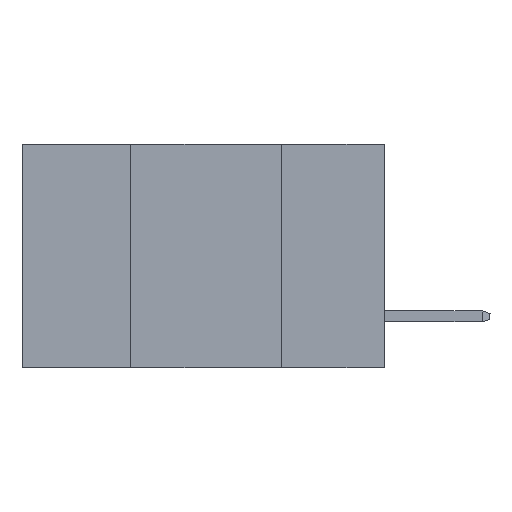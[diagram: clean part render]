
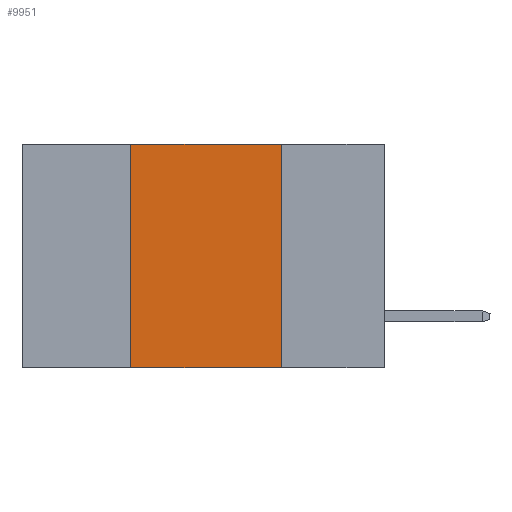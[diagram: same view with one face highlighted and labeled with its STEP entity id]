
A CAD part, left-side view. The second image highlights one B-rep face of the part: STEP entity #9951.
In plain terms, the highlighted planar face has unit normal (-1, 0, 0).
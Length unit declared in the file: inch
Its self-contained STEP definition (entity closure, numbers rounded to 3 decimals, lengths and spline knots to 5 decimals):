
#130 = CARTESIAN_POINT ( 'NONE',  ( 0., 0.17, -0.37 ) ) ;
#491 = DIRECTION ( 'NONE',  ( 0., -1., 0. ) ) ;
#654 = DIRECTION ( 'NONE',  ( 0., 0., 1. ) ) ;
#1088 = VECTOR ( 'NONE', #7853, 39.37008 ) ;
#1345 = VECTOR ( 'NONE', #9363, 39.37008 ) ;
#1347 = VECTOR ( 'NONE', #491, 39.37008 ) ;
#1742 = LINE ( 'NONE', #5525, #1088 ) ;
#1953 = ORIENTED_EDGE ( 'NONE', *, *, #2191, .F. ) ;
#2119 = EDGE_CURVE ( 'NONE', #2372, #7838, #6207, .T. ) ;
#2191 = EDGE_CURVE ( 'NONE', #3699, #8662, #4526, .T. ) ;
#2372 = VERTEX_POINT ( 'NONE', #8064 ) ;
#2835 = CARTESIAN_POINT ( 'NONE',  ( 0., 0.6, -0.37 ) ) ;
#3263 = VECTOR ( 'NONE', #654, 39.37008 ) ;
#3496 = CARTESIAN_POINT ( 'NONE',  ( 0., 0.42, -0.37 ) ) ;
#3699 = VERTEX_POINT ( 'NONE', #3496 ) ;
#3787 = FACE_OUTER_BOUND ( 'NONE', #6253, .T. ) ;
#4526 = LINE ( 'NONE', #7595, #3263 ) ;
#4546 = CARTESIAN_POINT ( 'NONE',  ( 0., 0.6, 0. ) ) ;
#5272 = EDGE_CURVE ( 'NONE', #8662, #2372, #1742, .T. ) ;
#5525 = CARTESIAN_POINT ( 'NONE',  ( 0., 0.6, 0. ) ) ;
#5648 = DIRECTION ( 'NONE',  ( 0., 0., -1. ) ) ;
#6035 = DIRECTION ( 'NONE',  ( 1., 0., 0. ) ) ;
#6207 = LINE ( 'NONE', #6247, #1345 ) ;
#6247 = CARTESIAN_POINT ( 'NONE',  ( 0., 0.17, -0.37 ) ) ;
#6253 = EDGE_LOOP ( 'NONE', ( #8322, #9715, #1953, #6516 ) ) ;
#6516 = ORIENTED_EDGE ( 'NONE', *, *, #7517, .T. ) ;
#6659 = LINE ( 'NONE', #2835, #1347 ) ;
#7517 = EDGE_CURVE ( 'NONE', #3699, #7838, #6659, .T. ) ;
#7595 = CARTESIAN_POINT ( 'NONE',  ( 0., 0.42, -0.37 ) ) ;
#7838 = VERTEX_POINT ( 'NONE', #130 ) ;
#7853 = DIRECTION ( 'NONE',  ( 0., -1., 0. ) ) ;
#7973 = AXIS2_PLACEMENT_3D ( 'NONE', #4546, #6035, #5648 ) ;
#8064 = CARTESIAN_POINT ( 'NONE',  ( 0., 0.17, 0. ) ) ;
#8322 = ORIENTED_EDGE ( 'NONE', *, *, #2119, .F. ) ;
#8662 = VERTEX_POINT ( 'NONE', #9474 ) ;
#9363 = DIRECTION ( 'NONE',  ( 0., 0., -1. ) ) ;
#9474 = CARTESIAN_POINT ( 'NONE',  ( 0., 0.42, 0. ) ) ;
#9715 = ORIENTED_EDGE ( 'NONE', *, *, #5272, .F. ) ;
#9951 = ADVANCED_FACE ( 'NONE', ( #3787 ), #9954, .F. ) ;
#9954 = PLANE ( 'NONE',  #7973 ) ;
